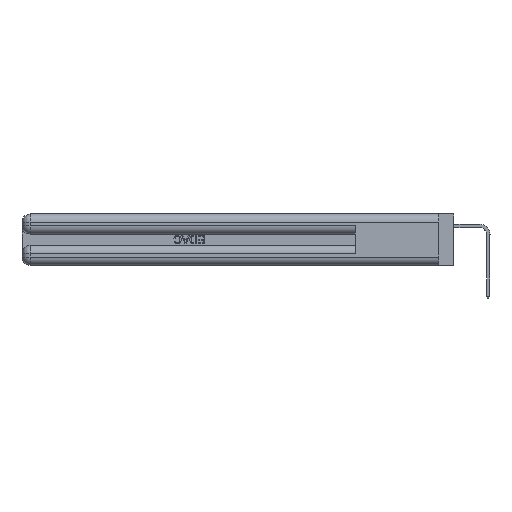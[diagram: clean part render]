
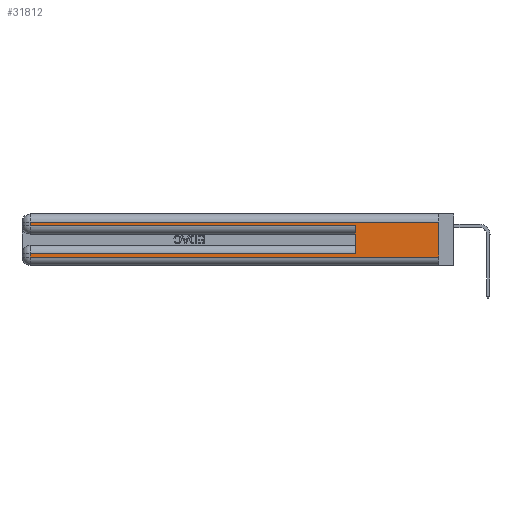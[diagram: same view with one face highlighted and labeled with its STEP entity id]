
A CAD part, left-side view. The second image highlights one B-rep face of the part: STEP entity #31812.
In plain terms, the highlighted planar face has unit normal (-1, 0, 0).
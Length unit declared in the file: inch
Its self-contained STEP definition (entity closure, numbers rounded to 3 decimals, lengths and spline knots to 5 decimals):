
#246 = EDGE_CURVE ( 'NONE', #2314, #9897, #35931, .T. ) ;
#339 = DIRECTION ( 'NONE',  ( 0., 0., -1. ) ) ;
#623 = LINE ( 'NONE', #11246, #25340 ) ;
#1711 = CARTESIAN_POINT ( 'NONE',  ( 0., 0.6, 0.285 ) ) ;
#2314 = VERTEX_POINT ( 'NONE', #8261 ) ;
#3318 = CARTESIAN_POINT ( 'NONE',  ( 0., 0., 0.37 ) ) ;
#3465 = ORIENTED_EDGE ( 'NONE', *, *, #246, .F. ) ;
#3665 = VERTEX_POINT ( 'NONE', #1711 ) ;
#4045 = VECTOR ( 'NONE', #24848, 39.37008 ) ;
#5049 = LINE ( 'NONE', #40783, #4045 ) ;
#5374 = EDGE_CURVE ( 'NONE', #27656, #22563, #29455, .T. ) ;
#5918 = LINE ( 'NONE', #21809, #13514 ) ;
#6839 = CARTESIAN_POINT ( 'NONE',  ( 0., 2.94, 0.06 ) ) ;
#8186 = EDGE_LOOP ( 'NONE', ( #3465, #40168, #17085, #16553, #27615, #21047, #33083, #26457 ) ) ;
#8189 = CARTESIAN_POINT ( 'NONE',  ( 0., 0.6, 0.145 ) ) ;
#8261 = CARTESIAN_POINT ( 'NONE',  ( 0., 0., 0.31 ) ) ;
#9748 = LINE ( 'NONE', #18686, #18351 ) ;
#9806 = DIRECTION ( 'NONE',  ( 0., 0., -1. ) ) ;
#9897 = VERTEX_POINT ( 'NONE', #31502 ) ;
#10290 = VECTOR ( 'NONE', #9806, 39.37008 ) ;
#11246 = CARTESIAN_POINT ( 'NONE',  ( 0., 0., 0.06 ) ) ;
#11766 = CARTESIAN_POINT ( 'NONE',  ( 0., 2.94, 0.085 ) ) ;
#12156 = PLANE ( 'NONE',  #30209 ) ;
#12354 = DIRECTION ( 'NONE',  ( 0., -1., 0. ) ) ;
#13514 = VECTOR ( 'NONE', #40985, 39.37008 ) ;
#13815 = LINE ( 'NONE', #29252, #38405 ) ;
#14507 = DIRECTION ( 'NONE',  ( 0., -1., 0. ) ) ;
#14722 = DIRECTION ( 'NONE',  ( 0., 0., 1. ) ) ;
#15405 = VECTOR ( 'NONE', #14722, 39.37008 ) ;
#16192 = EDGE_CURVE ( 'NONE', #27656, #3665, #40977, .T. ) ;
#16553 = ORIENTED_EDGE ( 'NONE', *, *, #22682, .T. ) ;
#17085 = ORIENTED_EDGE ( 'NONE', *, *, #29155, .T. ) ;
#17119 = CARTESIAN_POINT ( 'NONE',  ( 0., 0.6, 0.085 ) ) ;
#18351 = VECTOR ( 'NONE', #12354, 39.37008 ) ;
#18648 = DIRECTION ( 'NONE',  ( 0., 0., -1. ) ) ;
#18686 = CARTESIAN_POINT ( 'NONE',  ( 0., 0., 0.285 ) ) ;
#20877 = VECTOR ( 'NONE', #36449, 39.37008 ) ;
#21047 = ORIENTED_EDGE ( 'NONE', *, *, #5374, .T. ) ;
#21809 = CARTESIAN_POINT ( 'NONE',  ( 0., 2.94, 0.37 ) ) ;
#22563 = VERTEX_POINT ( 'NONE', #11766 ) ;
#22682 = EDGE_CURVE ( 'NONE', #39490, #3665, #9748, .T. ) ;
#24848 = DIRECTION ( 'NONE',  ( 0., 1., 0. ) ) ;
#25340 = VECTOR ( 'NONE', #14507, 39.37008 ) ;
#25637 = EDGE_CURVE ( 'NONE', #37150, #9897, #623, .T. ) ;
#26457 = ORIENTED_EDGE ( 'NONE', *, *, #25637, .T. ) ;
#27615 = ORIENTED_EDGE ( 'NONE', *, *, #16192, .F. ) ;
#27656 = VERTEX_POINT ( 'NONE', #17119 ) ;
#29155 = EDGE_CURVE ( 'NONE', #37827, #39490, #5918, .T. ) ;
#29252 = CARTESIAN_POINT ( 'NONE',  ( 0., 2.94, 0.37 ) ) ;
#29455 = LINE ( 'NONE', #33253, #20877 ) ;
#30209 = AXIS2_PLACEMENT_3D ( 'NONE', #34632, #37846, #18648 ) ;
#31176 = CARTESIAN_POINT ( 'NONE',  ( 0., 2.94, 0.31 ) ) ;
#31502 = CARTESIAN_POINT ( 'NONE',  ( 0., 0., 0.06 ) ) ;
#31812 = ADVANCED_FACE ( 'NONE', ( #39879 ), #12156, .F. ) ;
#32085 = EDGE_CURVE ( 'NONE', #22563, #37150, #13815, .T. ) ;
#33083 = ORIENTED_EDGE ( 'NONE', *, *, #32085, .T. ) ;
#33253 = CARTESIAN_POINT ( 'NONE',  ( 0., 0., 0.085 ) ) ;
#34632 = CARTESIAN_POINT ( 'NONE',  ( 0., 0., 0.37 ) ) ;
#35931 = LINE ( 'NONE', #3318, #10290 ) ;
#35935 = CARTESIAN_POINT ( 'NONE',  ( 0., 2.94, 0.285 ) ) ;
#36449 = DIRECTION ( 'NONE',  ( 0., 1., 0. ) ) ;
#37150 = VERTEX_POINT ( 'NONE', #6839 ) ;
#37827 = VERTEX_POINT ( 'NONE', #31176 ) ;
#37846 = DIRECTION ( 'NONE',  ( 1., 0., 0. ) ) ;
#38405 = VECTOR ( 'NONE', #339, 39.37008 ) ;
#39490 = VERTEX_POINT ( 'NONE', #35935 ) ;
#39843 = EDGE_CURVE ( 'NONE', #2314, #37827, #5049, .T. ) ;
#39879 = FACE_OUTER_BOUND ( 'NONE', #8186, .T. ) ;
#40168 = ORIENTED_EDGE ( 'NONE', *, *, #39843, .T. ) ;
#40783 = CARTESIAN_POINT ( 'NONE',  ( 0., 0., 0.31 ) ) ;
#40977 = LINE ( 'NONE', #8189, #15405 ) ;
#40985 = DIRECTION ( 'NONE',  ( 0., 0., -1. ) ) ;
